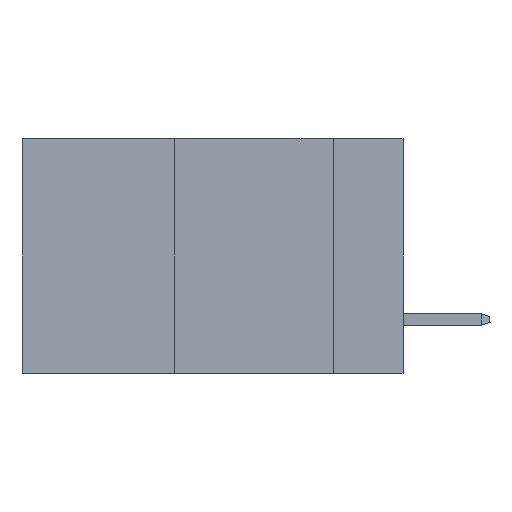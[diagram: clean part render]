
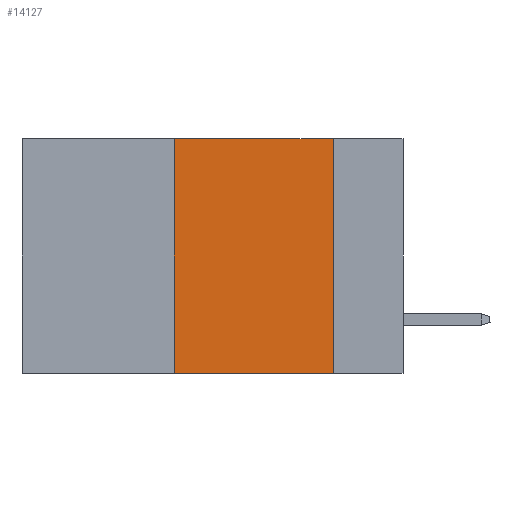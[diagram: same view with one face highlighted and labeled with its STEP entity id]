
A CAD part, left-side view. The second image highlights one B-rep face of the part: STEP entity #14127.
In plain terms, the highlighted planar face has unit normal (-1, 0, 0).
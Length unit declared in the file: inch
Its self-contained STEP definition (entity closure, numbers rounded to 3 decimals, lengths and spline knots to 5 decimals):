
#59 = EDGE_LOOP ( 'NONE', ( #3399, #7214, #14105, #12681 ) ) ;
#243 = CARTESIAN_POINT ( 'NONE',  ( 0., 0.11, 0. ) ) ;
#1433 = EDGE_CURVE ( 'NONE', #7236, #19351, #15138, .T. ) ;
#1847 = CARTESIAN_POINT ( 'NONE',  ( 0., 0.6, 0. ) ) ;
#1891 = DIRECTION ( 'NONE',  ( 0., -1., 0. ) ) ;
#2674 = EDGE_CURVE ( 'NONE', #12814, #14182, #13589, .T. ) ;
#3169 = LINE ( 'NONE', #9174, #15268 ) ;
#3399 = ORIENTED_EDGE ( 'NONE', *, *, #1433, .F. ) ;
#3418 = FACE_OUTER_BOUND ( 'NONE', #59, .T. ) ;
#4182 = CARTESIAN_POINT ( 'NONE',  ( 0., 0.11, -0.37 ) ) ;
#4474 = DIRECTION ( 'NONE',  ( 0., -1., 0. ) ) ;
#4955 = DIRECTION ( 'NONE',  ( 0., 0., -1. ) ) ;
#6364 = VECTOR ( 'NONE', #4474, 39.37008 ) ;
#6376 = DIRECTION ( 'NONE',  ( 1., 0., 0. ) ) ;
#7214 = ORIENTED_EDGE ( 'NONE', *, *, #16968, .F. ) ;
#7236 = VERTEX_POINT ( 'NONE', #7501 ) ;
#7468 = EDGE_CURVE ( 'NONE', #12814, #19351, #3169, .T. ) ;
#7501 = CARTESIAN_POINT ( 'NONE',  ( 0., 0.11, 0. ) ) ;
#7750 = PLANE ( 'NONE',  #9762 ) ;
#9174 = CARTESIAN_POINT ( 'NONE',  ( 0., 0.6, -0.37 ) ) ;
#9514 = CARTESIAN_POINT ( 'NONE',  ( 0., 0.36, 0. ) ) ;
#9762 = AXIS2_PLACEMENT_3D ( 'NONE', #1847, #6376, #13511 ) ;
#10749 = CARTESIAN_POINT ( 'NONE',  ( 0., 0.36, 0. ) ) ;
#11721 = VECTOR ( 'NONE', #4955, 39.37008 ) ;
#11842 = CARTESIAN_POINT ( 'NONE',  ( 0., 0.6, 0. ) ) ;
#12681 = ORIENTED_EDGE ( 'NONE', *, *, #7468, .T. ) ;
#12814 = VERTEX_POINT ( 'NONE', #18493 ) ;
#13511 = DIRECTION ( 'NONE',  ( 0., 0., -1. ) ) ;
#13589 = LINE ( 'NONE', #10749, #16792 ) ;
#14105 = ORIENTED_EDGE ( 'NONE', *, *, #2674, .F. ) ;
#14127 = ADVANCED_FACE ( 'NONE', ( #3418 ), #7750, .F. ) ;
#14182 = VERTEX_POINT ( 'NONE', #9514 ) ;
#14941 = DIRECTION ( 'NONE',  ( 0., 0., 1. ) ) ;
#15138 = LINE ( 'NONE', #243, #11721 ) ;
#15268 = VECTOR ( 'NONE', #1891, 39.37008 ) ;
#16142 = LINE ( 'NONE', #11842, #6364 ) ;
#16792 = VECTOR ( 'NONE', #14941, 39.37008 ) ;
#16968 = EDGE_CURVE ( 'NONE', #14182, #7236, #16142, .T. ) ;
#18493 = CARTESIAN_POINT ( 'NONE',  ( 0., 0.36, -0.37 ) ) ;
#19351 = VERTEX_POINT ( 'NONE', #4182 ) ;
